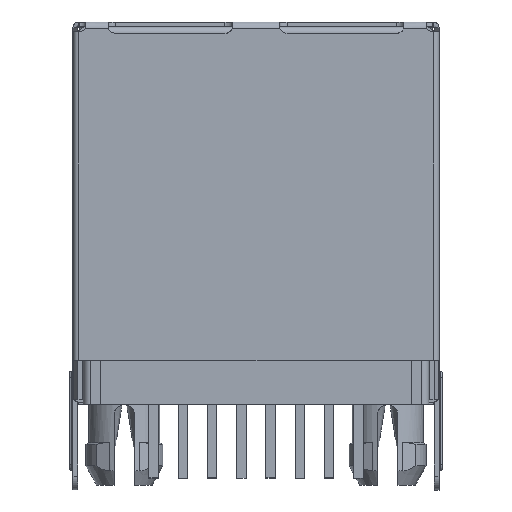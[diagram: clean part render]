
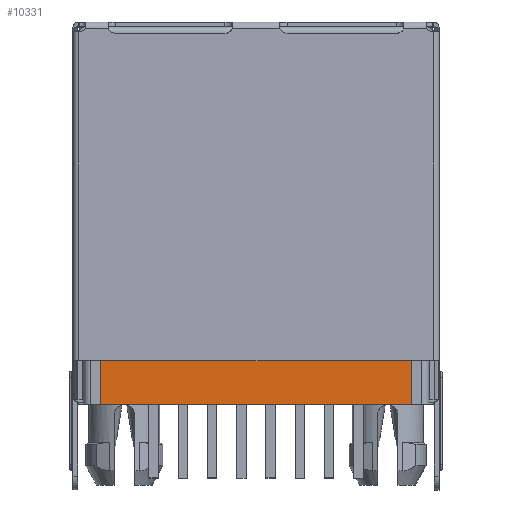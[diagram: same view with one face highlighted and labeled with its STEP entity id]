
A CAD part, top view. The second image highlights one B-rep face of the part: STEP entity #10331.
In plain terms, the highlighted planar face has unit normal (0, 0, 1).
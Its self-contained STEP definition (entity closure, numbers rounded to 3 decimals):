
#810 = CARTESIAN_POINT ( 'NONE',  ( 6.75, -16.4, 9.95 ) ) ;
#2134 = LINE ( 'NONE', #15867, #24789 ) ;
#2306 = LINE ( 'NONE', #14353, #6880 ) ;
#3690 = CARTESIAN_POINT ( 'NONE',  ( 6.75, -16.4, 9.95 ) ) ;
#5743 = FACE_OUTER_BOUND ( 'NONE', #9615, .T. ) ;
#6724 = VERTEX_POINT ( 'NONE', #36057 ) ;
#6880 = VECTOR ( 'NONE', #29230, 1000. ) ;
#9355 = EDGE_CURVE ( 'NONE', #10698, #6724, #31904, .T. ) ;
#9615 = EDGE_LOOP ( 'NONE', ( #14152, #33282, #22474, #25526 ) ) ;
#10331 = ADVANCED_FACE ( 'NONE', ( #5743 ), #13580, .T. ) ;
#10698 = VERTEX_POINT ( 'NONE', #11745 ) ;
#11745 = CARTESIAN_POINT ( 'NONE',  ( 6.75, -2.9, 9.95 ) ) ;
#13453 = CARTESIAN_POINT ( 'NONE',  ( 6.75, -2.9, 9.95 ) ) ;
#13580 = PLANE ( 'NONE',  #25583 ) ;
#14152 = ORIENTED_EDGE ( 'NONE', *, *, #25030, .T. ) ;
#14353 = CARTESIAN_POINT ( 'NONE',  ( 6.75, -2.9, 9.95 ) ) ;
#15867 = CARTESIAN_POINT ( 'NONE',  ( -6.75, -2.9, 9.95 ) ) ;
#18428 = EDGE_CURVE ( 'NONE', #30171, #29488, #32750, .T. ) ;
#19665 = DIRECTION ( 'NONE',  ( 1., 0., 0. ) ) ;
#22212 = CARTESIAN_POINT ( 'NONE',  ( -6.75, -16.4, 9.95 ) ) ;
#22474 = ORIENTED_EDGE ( 'NONE', *, *, #33476, .T. ) ;
#22799 = DIRECTION ( 'NONE',  ( 0., 0., 1. ) ) ;
#23146 = DIRECTION ( 'NONE',  ( -1., 0., 0. ) ) ;
#24789 = VECTOR ( 'NONE', #27906, 1000. ) ;
#25030 = EDGE_CURVE ( 'NONE', #29488, #10698, #2306, .T. ) ;
#25526 = ORIENTED_EDGE ( 'NONE', *, *, #18428, .T. ) ;
#25583 = AXIS2_PLACEMENT_3D ( 'NONE', #13453, #22799, #19665 ) ;
#25830 = CARTESIAN_POINT ( 'NONE',  ( 6.75, -2.9, 9.95 ) ) ;
#27254 = VECTOR ( 'NONE', #23146, 1000. ) ;
#27350 = DIRECTION ( 'NONE',  ( 1., 0., 0. ) ) ;
#27906 = DIRECTION ( 'NONE',  ( 0., -1., 0. ) ) ;
#29230 = DIRECTION ( 'NONE',  ( 0., 1., 0. ) ) ;
#29488 = VERTEX_POINT ( 'NONE', #810 ) ;
#30171 = VERTEX_POINT ( 'NONE', #22212 ) ;
#31904 = LINE ( 'NONE', #25830, #27254 ) ;
#32750 = LINE ( 'NONE', #3690, #37850 ) ;
#33282 = ORIENTED_EDGE ( 'NONE', *, *, #9355, .T. ) ;
#33476 = EDGE_CURVE ( 'NONE', #6724, #30171, #2134, .T. ) ;
#36057 = CARTESIAN_POINT ( 'NONE',  ( -6.75, -2.9, 9.95 ) ) ;
#37850 = VECTOR ( 'NONE', #27350, 1000. ) ;
